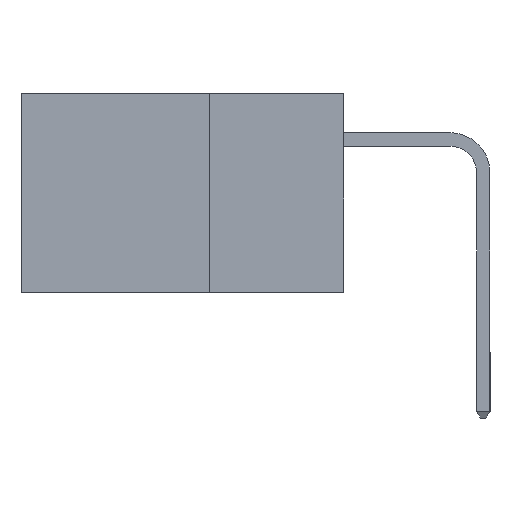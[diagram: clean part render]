
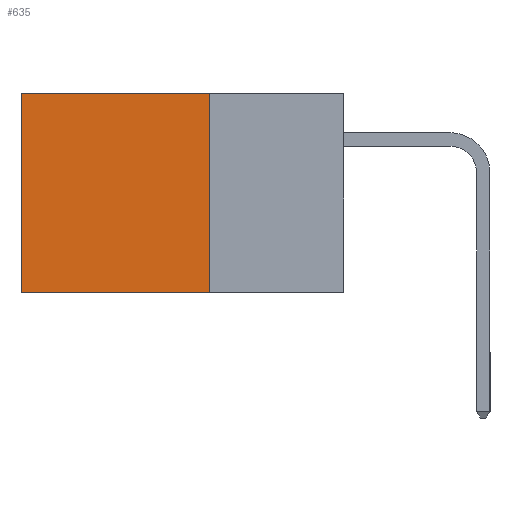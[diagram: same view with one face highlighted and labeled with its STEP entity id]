
A CAD part, left-side view. The second image highlights one B-rep face of the part: STEP entity #635.
In plain terms, the highlighted planar face has unit normal (-1, 0, 0).
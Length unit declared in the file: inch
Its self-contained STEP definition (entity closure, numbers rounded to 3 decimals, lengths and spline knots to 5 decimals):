
#635 = ADVANCED_FACE ( 'NONE', ( #10744 ), #693, .F. ) ;
#693 = PLANE ( 'NONE',  #8730 ) ;
#790 = ORIENTED_EDGE ( 'NONE', *, *, #10304, .T. ) ;
#847 = CARTESIAN_POINT ( 'NONE',  ( 0.2615, 0.25, -0.37 ) ) ;
#1180 = VECTOR ( 'NONE', #13408, 39.37008 ) ;
#1218 = ORIENTED_EDGE ( 'NONE', *, *, #1996, .T. ) ;
#1381 = LINE ( 'NONE', #14052, #13302 ) ;
#1695 = ORIENTED_EDGE ( 'NONE', *, *, #4931, .F. ) ;
#1996 = EDGE_CURVE ( 'NONE', #6322, #7740, #2560, .T. ) ;
#2035 = CARTESIAN_POINT ( 'NONE',  ( 0.2615, 0.25, 0. ) ) ;
#2046 = CARTESIAN_POINT ( 'NONE',  ( 0.2615, 0.25, 0. ) ) ;
#2560 = LINE ( 'NONE', #8596, #7663 ) ;
#3157 = EDGE_LOOP ( 'NONE', ( #1218, #1695, #13685, #790 ) ) ;
#4349 = DIRECTION ( 'NONE',  ( 0., 0., -1. ) ) ;
#4931 = EDGE_CURVE ( 'NONE', #9245, #7740, #10882, .T. ) ;
#5791 = DIRECTION ( 'NONE',  ( 0., 1., 0. ) ) ;
#6286 = CARTESIAN_POINT ( 'NONE',  ( 0.2615, 0.6, 0. ) ) ;
#6291 = VERTEX_POINT ( 'NONE', #2046 ) ;
#6322 = VERTEX_POINT ( 'NONE', #6286 ) ;
#6523 = DIRECTION ( 'NONE',  ( 0., 0., -1. ) ) ;
#6963 = DIRECTION ( 'NONE',  ( 1., 0., 0. ) ) ;
#7155 = CARTESIAN_POINT ( 'NONE',  ( 0.2615, 0.6, -0.37 ) ) ;
#7663 = VECTOR ( 'NONE', #15967, 39.37008 ) ;
#7740 = VERTEX_POINT ( 'NONE', #7155 ) ;
#8596 = CARTESIAN_POINT ( 'NONE',  ( 0.2615, 0.6, -0.37 ) ) ;
#8730 = AXIS2_PLACEMENT_3D ( 'NONE', #847, #6963, #4349 ) ;
#9245 = VERTEX_POINT ( 'NONE', #15185 ) ;
#10304 = EDGE_CURVE ( 'NONE', #6291, #6322, #10872, .T. ) ;
#10744 = FACE_OUTER_BOUND ( 'NONE', #3157, .T. ) ;
#10872 = LINE ( 'NONE', #2035, #15599 ) ;
#10882 = LINE ( 'NONE', #15527, #1180 ) ;
#11771 = EDGE_CURVE ( 'NONE', #6291, #9245, #1381, .T. ) ;
#13302 = VECTOR ( 'NONE', #6523, 39.37008 ) ;
#13408 = DIRECTION ( 'NONE',  ( 0., 1., 0. ) ) ;
#13685 = ORIENTED_EDGE ( 'NONE', *, *, #11771, .F. ) ;
#14052 = CARTESIAN_POINT ( 'NONE',  ( 0.2615, 0.25, -0.37 ) ) ;
#15185 = CARTESIAN_POINT ( 'NONE',  ( 0.2615, 0.25, -0.37 ) ) ;
#15527 = CARTESIAN_POINT ( 'NONE',  ( 0.2615, 0.25, -0.37 ) ) ;
#15599 = VECTOR ( 'NONE', #5791, 39.37008 ) ;
#15967 = DIRECTION ( 'NONE',  ( 0., 0., -1. ) ) ;
